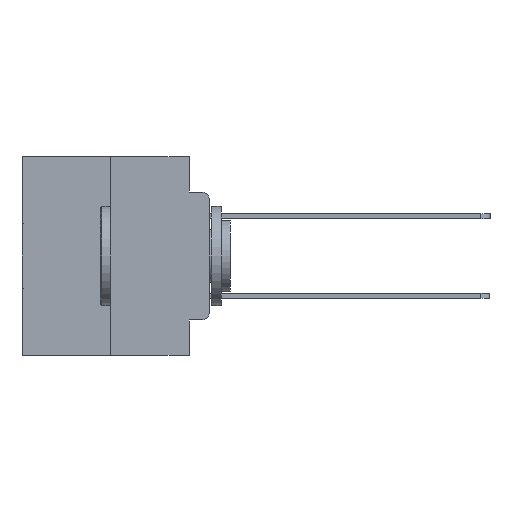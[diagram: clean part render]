
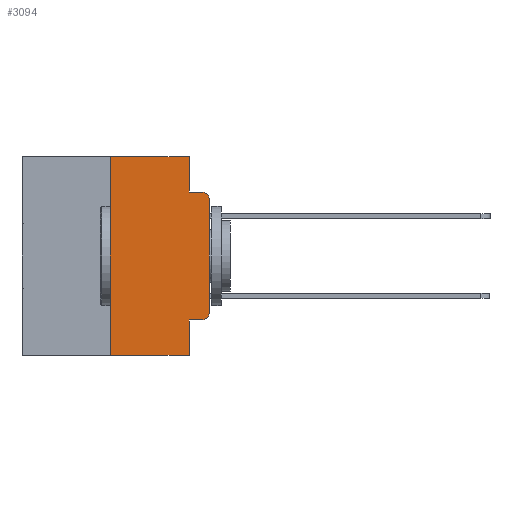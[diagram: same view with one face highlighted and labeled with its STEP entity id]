
A CAD part, left-side view. The second image highlights one B-rep face of the part: STEP entity #3094.
In plain terms, the highlighted planar face has unit normal (-1, 0, 0).
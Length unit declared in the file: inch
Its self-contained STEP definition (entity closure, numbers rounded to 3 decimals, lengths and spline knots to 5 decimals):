
#33 = VERTEX_POINT ( 'NONE', #12363 ) ;
#120 = EDGE_CURVE ( 'NONE', #26343, #19137, #24368, .T. ) ;
#568 = EDGE_LOOP ( 'NONE', ( #25918, #8685, #21186, #21915, #10161, #16416, #17171, #29486, #12386, #581 ) ) ;
#581 = ORIENTED_EDGE ( 'NONE', *, *, #19682, .T. ) ;
#809 = EDGE_CURVE ( 'NONE', #26015, #19137, #24691, .T. ) ;
#1152 = LINE ( 'NONE', #8178, #12942 ) ;
#1332 = VECTOR ( 'NONE', #13956, 39.37008 ) ;
#1408 = VERTEX_POINT ( 'NONE', #5077 ) ;
#2669 = DIRECTION ( 'NONE',  ( 0., 0., 1. ) ) ;
#2765 = EDGE_CURVE ( 'NONE', #20042, #9478, #30154, .T. ) ;
#2770 = CARTESIAN_POINT ( 'NONE',  ( 0., 0.25, 0. ) ) ;
#3094 = ADVANCED_FACE ( 'NONE', ( #24429 ), #14379, .F. ) ;
#3235 = CARTESIAN_POINT ( 'NONE',  ( 0., 0., -0.3915 ) ) ;
#3633 = AXIS2_PLACEMENT_3D ( 'NONE', #4741, #21167, #7104 ) ;
#3640 = AXIS2_PLACEMENT_3D ( 'NONE', #13298, #29567, #15661 ) ;
#4505 = CARTESIAN_POINT ( 'NONE',  ( 0., 0., 0. ) ) ;
#4741 = CARTESIAN_POINT ( 'NONE',  ( 0., 0.02, -0.3915 ) ) ;
#4867 = CARTESIAN_POINT ( 'NONE',  ( 0., 0.051, 0. ) ) ;
#5062 = DIRECTION ( 'NONE',  ( 0., 0., -1. ) ) ;
#5077 = CARTESIAN_POINT ( 'NONE',  ( 0., 0.02, -0.0885 ) ) ;
#5364 = VECTOR ( 'NONE', #24345, 39.37008 ) ;
#6163 = CARTESIAN_POINT ( 'NONE',  ( 0., 0.051, 0. ) ) ;
#6991 = VERTEX_POINT ( 'NONE', #3235 ) ;
#7104 = DIRECTION ( 'NONE',  ( 0., 0., -1. ) ) ;
#7313 = VECTOR ( 'NONE', #14593, 39.37008 ) ;
#7475 = EDGE_CURVE ( 'NONE', #9478, #1408, #19809, .T. ) ;
#8178 = CARTESIAN_POINT ( 'NONE',  ( 0., 0.473, 0. ) ) ;
#8607 = CIRCLE ( 'NONE', #3633, 0.02 ) ;
#8685 = ORIENTED_EDGE ( 'NONE', *, *, #9036, .T. ) ;
#9036 = EDGE_CURVE ( 'NONE', #16854, #1408, #11413, .T. ) ;
#9478 = VERTEX_POINT ( 'NONE', #15223 ) ;
#9758 = DIRECTION ( 'NONE',  ( 0., -1., 0. ) ) ;
#10161 = ORIENTED_EDGE ( 'NONE', *, *, #25214, .F. ) ;
#10530 = DIRECTION ( 'NONE',  ( 0., -1., 0. ) ) ;
#11413 = CIRCLE ( 'NONE', #3640, 0.02 ) ;
#12219 = EDGE_CURVE ( 'NONE', #6991, #16854, #25557, .T. ) ;
#12255 = CARTESIAN_POINT ( 'NONE',  ( 0., 0., -0.1085 ) ) ;
#12363 = CARTESIAN_POINT ( 'NONE',  ( 0., 0.25, 0. ) ) ;
#12386 = ORIENTED_EDGE ( 'NONE', *, *, #24363, .T. ) ;
#12942 = VECTOR ( 'NONE', #10530, 39.37008 ) ;
#13015 = CARTESIAN_POINT ( 'NONE',  ( 0., 0.02, -0.4115 ) ) ;
#13298 = CARTESIAN_POINT ( 'NONE',  ( 0., 0.02, -0.1085 ) ) ;
#13956 = DIRECTION ( 'NONE',  ( 0., 0., 1. ) ) ;
#14345 = CARTESIAN_POINT ( 'NONE',  ( 0., 0.473, 0. ) ) ;
#14379 = PLANE ( 'NONE',  #24228 ) ;
#14593 = DIRECTION ( 'NONE',  ( 0., -1., 0. ) ) ;
#15223 = CARTESIAN_POINT ( 'NONE',  ( 0., 0.051, -0.0885 ) ) ;
#15661 = DIRECTION ( 'NONE',  ( 0., 0., -1. ) ) ;
#15711 = CARTESIAN_POINT ( 'NONE',  ( 0., 0.051, -0.5 ) ) ;
#16416 = ORIENTED_EDGE ( 'NONE', *, *, #28402, .F. ) ;
#16578 = DIRECTION ( 'NONE',  ( 0., 0., -1. ) ) ;
#16588 = DIRECTION ( 'NONE',  ( 1., 0., 0. ) ) ;
#16854 = VERTEX_POINT ( 'NONE', #12255 ) ;
#17171 = ORIENTED_EDGE ( 'NONE', *, *, #809, .T. ) ;
#17728 = VERTEX_POINT ( 'NONE', #13015 ) ;
#18474 = VECTOR ( 'NONE', #19760, 39.37008 ) ;
#19137 = VERTEX_POINT ( 'NONE', #15711 ) ;
#19682 = EDGE_CURVE ( 'NONE', #17728, #6991, #8607, .T. ) ;
#19760 = DIRECTION ( 'NONE',  ( 0., -1., 0. ) ) ;
#19809 = LINE ( 'NONE', #28538, #7313 ) ;
#20042 = VERTEX_POINT ( 'NONE', #6163 ) ;
#21167 = DIRECTION ( 'NONE',  ( -1., 0., 0. ) ) ;
#21186 = ORIENTED_EDGE ( 'NONE', *, *, #7475, .F. ) ;
#21208 = CARTESIAN_POINT ( 'NONE',  ( 0., 0.473, -0.5 ) ) ;
#21479 = LINE ( 'NONE', #23795, #22204 ) ;
#21915 = ORIENTED_EDGE ( 'NONE', *, *, #2765, .F. ) ;
#22204 = VECTOR ( 'NONE', #9758, 39.37008 ) ;
#23795 = CARTESIAN_POINT ( 'NONE',  ( 0., 0.051, -0.4115 ) ) ;
#24228 = AXIS2_PLACEMENT_3D ( 'NONE', #14345, #16588, #16578 ) ;
#24345 = DIRECTION ( 'NONE',  ( 0., 0., -1. ) ) ;
#24363 = EDGE_CURVE ( 'NONE', #26343, #17728, #21479, .T. ) ;
#24368 = LINE ( 'NONE', #4867, #29749 ) ;
#24429 = FACE_OUTER_BOUND ( 'NONE', #568, .T. ) ;
#24691 = LINE ( 'NONE', #21208, #18474 ) ;
#25032 = VECTOR ( 'NONE', #2669, 39.37008 ) ;
#25214 = EDGE_CURVE ( 'NONE', #33, #20042, #1152, .T. ) ;
#25444 = CARTESIAN_POINT ( 'NONE',  ( 0., 0.051, 0. ) ) ;
#25557 = LINE ( 'NONE', #4505, #1332 ) ;
#25766 = LINE ( 'NONE', #2770, #25032 ) ;
#25918 = ORIENTED_EDGE ( 'NONE', *, *, #12219, .T. ) ;
#26015 = VERTEX_POINT ( 'NONE', #29810 ) ;
#26343 = VERTEX_POINT ( 'NONE', #26413 ) ;
#26413 = CARTESIAN_POINT ( 'NONE',  ( 0., 0.051, -0.4115 ) ) ;
#28402 = EDGE_CURVE ( 'NONE', #26015, #33, #25766, .T. ) ;
#28538 = CARTESIAN_POINT ( 'NONE',  ( 0., 0.051, -0.0885 ) ) ;
#29486 = ORIENTED_EDGE ( 'NONE', *, *, #120, .F. ) ;
#29567 = DIRECTION ( 'NONE',  ( -1., 0., 0. ) ) ;
#29749 = VECTOR ( 'NONE', #5062, 39.37008 ) ;
#29810 = CARTESIAN_POINT ( 'NONE',  ( 0., 0.25, -0.5 ) ) ;
#30154 = LINE ( 'NONE', #25444, #5364 ) ;
